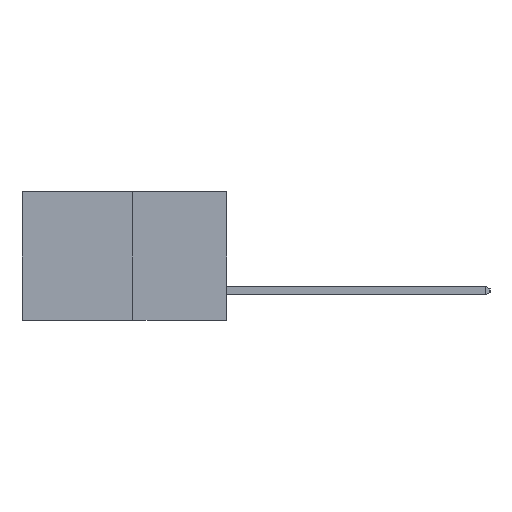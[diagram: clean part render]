
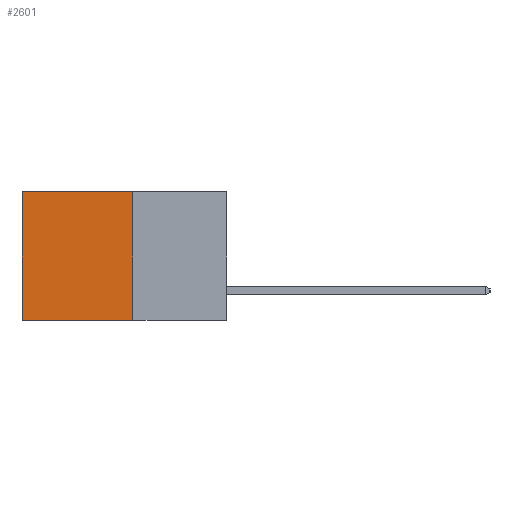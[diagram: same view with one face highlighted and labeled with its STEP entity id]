
A CAD part, left-side view. The second image highlights one B-rep face of the part: STEP entity #2601.
In plain terms, the highlighted planar face has unit normal (-1, 0, 0).
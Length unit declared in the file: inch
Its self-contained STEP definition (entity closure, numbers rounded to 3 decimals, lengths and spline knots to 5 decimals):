
#346 = CARTESIAN_POINT ( 'NONE',  ( 0.277, 0.27, 0. ) ) ;
#767 = DIRECTION ( 'NONE',  ( 0., 0., -1. ) ) ;
#1525 = VERTEX_POINT ( 'NONE', #12111 ) ;
#2226 = AXIS2_PLACEMENT_3D ( 'NONE', #4876, #18171, #767 ) ;
#2601 = ADVANCED_FACE ( 'NONE', ( #9311 ), #17000, .F. ) ;
#3104 = VECTOR ( 'NONE', #11106, 39.37008 ) ;
#3589 = EDGE_CURVE ( 'NONE', #16844, #1525, #7696, .T. ) ;
#3757 = CARTESIAN_POINT ( 'NONE',  ( 0.277, 0.59, 0. ) ) ;
#3889 = VERTEX_POINT ( 'NONE', #3757 ) ;
#4607 = DIRECTION ( 'NONE',  ( 0., 0., -1. ) ) ;
#4876 = CARTESIAN_POINT ( 'NONE',  ( 0.277, 0.27, -0.37 ) ) ;
#5199 = EDGE_CURVE ( 'NONE', #1525, #17069, #11845, .T. ) ;
#5260 = EDGE_CURVE ( 'NONE', #3889, #17069, #13719, .T. ) ;
#7060 = EDGE_LOOP ( 'NONE', ( #20040, #17684, #17986, #11314 ) ) ;
#7696 = LINE ( 'NONE', #12870, #22558 ) ;
#9311 = FACE_OUTER_BOUND ( 'NONE', #7060, .T. ) ;
#9580 = VECTOR ( 'NONE', #14458, 39.37008 ) ;
#10149 = VECTOR ( 'NONE', #12796, 39.37008 ) ;
#11106 = DIRECTION ( 'NONE',  ( 0., 1., 0. ) ) ;
#11314 = ORIENTED_EDGE ( 'NONE', *, *, #17008, .T. ) ;
#11845 = LINE ( 'NONE', #12954, #10149 ) ;
#12111 = CARTESIAN_POINT ( 'NONE',  ( 0.277, 0.27, -0.37 ) ) ;
#12796 = DIRECTION ( 'NONE',  ( 0., 1., 0. ) ) ;
#12870 = CARTESIAN_POINT ( 'NONE',  ( 0.277, 0.27, -0.37 ) ) ;
#12954 = CARTESIAN_POINT ( 'NONE',  ( 0.277, 0.27, -0.37 ) ) ;
#13719 = LINE ( 'NONE', #19361, #9580 ) ;
#14458 = DIRECTION ( 'NONE',  ( 0., 0., -1. ) ) ;
#16844 = VERTEX_POINT ( 'NONE', #22685 ) ;
#17000 = PLANE ( 'NONE',  #2226 ) ;
#17008 = EDGE_CURVE ( 'NONE', #16844, #3889, #17145, .T. ) ;
#17069 = VERTEX_POINT ( 'NONE', #19912 ) ;
#17145 = LINE ( 'NONE', #346, #3104 ) ;
#17684 = ORIENTED_EDGE ( 'NONE', *, *, #5199, .F. ) ;
#17986 = ORIENTED_EDGE ( 'NONE', *, *, #3589, .F. ) ;
#18171 = DIRECTION ( 'NONE',  ( 1., 0., 0. ) ) ;
#19361 = CARTESIAN_POINT ( 'NONE',  ( 0.277, 0.59, -0.37 ) ) ;
#19912 = CARTESIAN_POINT ( 'NONE',  ( 0.277, 0.59, -0.37 ) ) ;
#20040 = ORIENTED_EDGE ( 'NONE', *, *, #5260, .T. ) ;
#22558 = VECTOR ( 'NONE', #4607, 39.37008 ) ;
#22685 = CARTESIAN_POINT ( 'NONE',  ( 0.277, 0.27, 0. ) ) ;
